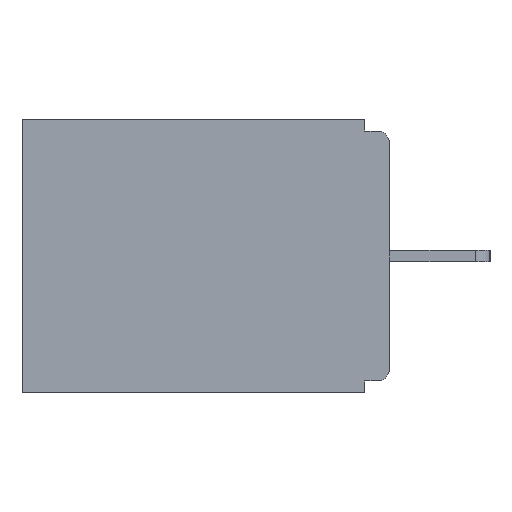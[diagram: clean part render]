
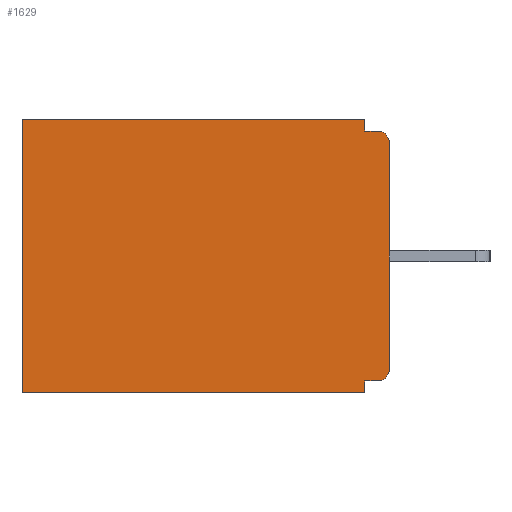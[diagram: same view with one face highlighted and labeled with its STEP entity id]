
A CAD part, left-side view. The second image highlights one B-rep face of the part: STEP entity #1629.
In plain terms, the highlighted planar face has unit normal (-1, 0, 0).
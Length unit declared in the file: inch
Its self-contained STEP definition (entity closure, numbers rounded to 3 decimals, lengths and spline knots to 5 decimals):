
#47 = DIRECTION ( 'NONE',  ( 0., 1., 0. ) ) ;
#80 = LINE ( 'NONE', #4033, #12974 ) ;
#603 = VERTEX_POINT ( 'NONE', #8627 ) ;
#636 = CARTESIAN_POINT ( 'NONE',  ( 0.298, 0.46, -0.343 ) ) ;
#668 = DIRECTION ( 'NONE',  ( 0., 0., -1. ) ) ;
#818 = ORIENTED_EDGE ( 'NONE', *, *, #11846, .T. ) ;
#899 = ORIENTED_EDGE ( 'NONE', *, *, #15371, .F. ) ;
#926 = CARTESIAN_POINT ( 'NONE',  ( 0.298, 0.015, -0.03 ) ) ;
#977 = CIRCLE ( 'NONE', #4405, 0.015 ) ;
#1087 = ORIENTED_EDGE ( 'NONE', *, *, #12349, .T. ) ;
#1480 = ORIENTED_EDGE ( 'NONE', *, *, #1813, .F. ) ;
#1593 = VECTOR ( 'NONE', #47, 39.37008 ) ;
#1629 = ADVANCED_FACE ( 'NONE', ( #9245 ), #1695, .F. ) ;
#1695 = PLANE ( 'NONE',  #13591 ) ;
#1813 = EDGE_CURVE ( 'NONE', #603, #14391, #4582, .T. ) ;
#2222 = EDGE_CURVE ( 'NONE', #14726, #3177, #14831, .T. ) ;
#2402 = DIRECTION ( 'NONE',  ( 0., 1., 0. ) ) ;
#2594 = AXIS2_PLACEMENT_3D ( 'NONE', #11564, #15153, #10017 ) ;
#3022 = LINE ( 'NONE', #13126, #8318 ) ;
#3177 = VERTEX_POINT ( 'NONE', #8803 ) ;
#3705 = VERTEX_POINT ( 'NONE', #636 ) ;
#3749 = DIRECTION ( 'NONE',  ( 0., 0., -1. ) ) ;
#4005 = CARTESIAN_POINT ( 'NONE',  ( 0.298, 0.031, -0.015 ) ) ;
#4033 = CARTESIAN_POINT ( 'NONE',  ( 0.298, 0., -0.328 ) ) ;
#4371 = VERTEX_POINT ( 'NONE', #7580 ) ;
#4405 = AXIS2_PLACEMENT_3D ( 'NONE', #926, #8527, #3749 ) ;
#4407 = ORIENTED_EDGE ( 'NONE', *, *, #2222, .F. ) ;
#4582 = LINE ( 'NONE', #9473, #6742 ) ;
#4868 = VECTOR ( 'NONE', #12901, 39.37008 ) ;
#4980 = VERTEX_POINT ( 'NONE', #9785 ) ;
#5083 = CARTESIAN_POINT ( 'NONE',  ( 0.298, 0.46, 0. ) ) ;
#5221 = CIRCLE ( 'NONE', #2594, 0.015 ) ;
#5323 = CARTESIAN_POINT ( 'NONE',  ( 0.298, 0., 0. ) ) ;
#5426 = DIRECTION ( 'NONE',  ( 0., 1., 0. ) ) ;
#5567 = EDGE_CURVE ( 'NONE', #14391, #4371, #12970, .T. ) ;
#6088 = EDGE_LOOP ( 'NONE', ( #818, #7985, #1480, #14921, #11397, #12146, #4407, #9505, #1087, #899 ) ) ;
#6742 = VECTOR ( 'NONE', #8388, 39.37008 ) ;
#7170 = EDGE_CURVE ( 'NONE', #3177, #3705, #12540, .T. ) ;
#7195 = CARTESIAN_POINT ( 'NONE',  ( 0.298, 0.46, 0. ) ) ;
#7580 = CARTESIAN_POINT ( 'NONE',  ( 0.298, 0.015, -0.015 ) ) ;
#7819 = DIRECTION ( 'NONE',  ( 1., 0., 0. ) ) ;
#7985 = ORIENTED_EDGE ( 'NONE', *, *, #5567, .F. ) ;
#8318 = VECTOR ( 'NONE', #5426, 39.37008 ) ;
#8388 = DIRECTION ( 'NONE',  ( 0., 0., -1. ) ) ;
#8527 = DIRECTION ( 'NONE',  ( -1., 0., 0. ) ) ;
#8627 = CARTESIAN_POINT ( 'NONE',  ( 0.298, 0.031, 0. ) ) ;
#8803 = CARTESIAN_POINT ( 'NONE',  ( 0.298, 0.031, -0.343 ) ) ;
#8871 = EDGE_CURVE ( 'NONE', #603, #12282, #3022, .T. ) ;
#9070 = CARTESIAN_POINT ( 'NONE',  ( 0.298, 0., 0. ) ) ;
#9245 = FACE_OUTER_BOUND ( 'NONE', #6088, .T. ) ;
#9473 = CARTESIAN_POINT ( 'NONE',  ( 0.298, 0.031, -0.343 ) ) ;
#9505 = ORIENTED_EDGE ( 'NONE', *, *, #15543, .F. ) ;
#9785 = CARTESIAN_POINT ( 'NONE',  ( 0.298, 0.015, -0.328 ) ) ;
#10017 = DIRECTION ( 'NONE',  ( 0., 0., -1. ) ) ;
#10201 = VECTOR ( 'NONE', #668, 39.37008 ) ;
#10290 = LINE ( 'NONE', #5323, #11884 ) ;
#10369 = DIRECTION ( 'NONE',  ( 0., 0., -1. ) ) ;
#11366 = LINE ( 'NONE', #5083, #14812 ) ;
#11397 = ORIENTED_EDGE ( 'NONE', *, *, #15281, .T. ) ;
#11564 = CARTESIAN_POINT ( 'NONE',  ( 0.298, 0.015, -0.313 ) ) ;
#11846 = EDGE_CURVE ( 'NONE', #12772, #4371, #977, .T. ) ;
#11884 = VECTOR ( 'NONE', #10369, 39.37008 ) ;
#12146 = ORIENTED_EDGE ( 'NONE', *, *, #7170, .F. ) ;
#12282 = VERTEX_POINT ( 'NONE', #7195 ) ;
#12349 = EDGE_CURVE ( 'NONE', #4980, #16302, #5221, .T. ) ;
#12540 = LINE ( 'NONE', #12711, #1593 ) ;
#12711 = CARTESIAN_POINT ( 'NONE',  ( 0.298, 0., -0.343 ) ) ;
#12772 = VERTEX_POINT ( 'NONE', #14181 ) ;
#12892 = DIRECTION ( 'NONE',  ( 0., 0., -1. ) ) ;
#12901 = DIRECTION ( 'NONE',  ( 0., -1., 0. ) ) ;
#12970 = LINE ( 'NONE', #14206, #4868 ) ;
#12974 = VECTOR ( 'NONE', #2402, 39.37008 ) ;
#13126 = CARTESIAN_POINT ( 'NONE',  ( 0.298, 0., 0. ) ) ;
#13591 = AXIS2_PLACEMENT_3D ( 'NONE', #9070, #7819, #12892 ) ;
#13981 = CARTESIAN_POINT ( 'NONE',  ( 0.298, 0.031, -0.328 ) ) ;
#14181 = CARTESIAN_POINT ( 'NONE',  ( 0.298, 0., -0.03 ) ) ;
#14206 = CARTESIAN_POINT ( 'NONE',  ( 0.298, 0., -0.015 ) ) ;
#14391 = VERTEX_POINT ( 'NONE', #4005 ) ;
#14726 = VERTEX_POINT ( 'NONE', #13981 ) ;
#14812 = VECTOR ( 'NONE', #15184, 39.37008 ) ;
#14831 = LINE ( 'NONE', #15989, #10201 ) ;
#14921 = ORIENTED_EDGE ( 'NONE', *, *, #8871, .T. ) ;
#15153 = DIRECTION ( 'NONE',  ( -1., 0., 0. ) ) ;
#15184 = DIRECTION ( 'NONE',  ( 0., 0., -1. ) ) ;
#15281 = EDGE_CURVE ( 'NONE', #12282, #3705, #11366, .T. ) ;
#15371 = EDGE_CURVE ( 'NONE', #12772, #16302, #10290, .T. ) ;
#15543 = EDGE_CURVE ( 'NONE', #4980, #14726, #80, .T. ) ;
#15989 = CARTESIAN_POINT ( 'NONE',  ( 0.298, 0.031, -0.343 ) ) ;
#16302 = VERTEX_POINT ( 'NONE', #16351 ) ;
#16351 = CARTESIAN_POINT ( 'NONE',  ( 0.298, 0., -0.313 ) ) ;
